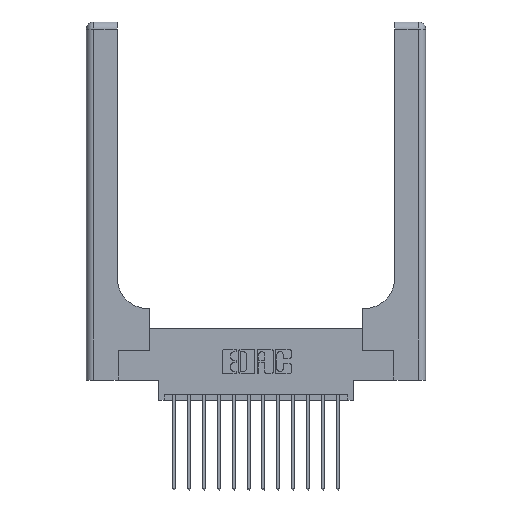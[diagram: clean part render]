
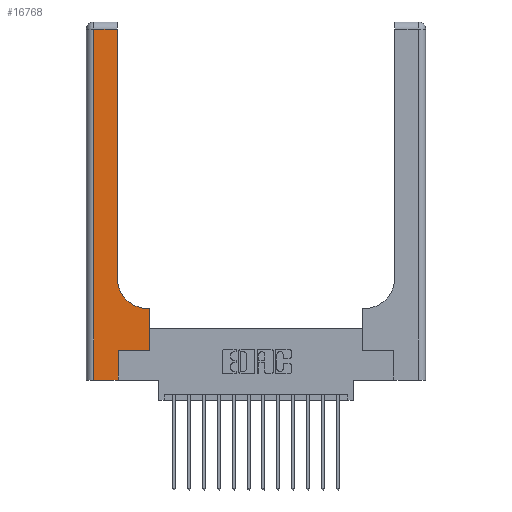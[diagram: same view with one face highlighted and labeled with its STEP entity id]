
A CAD part, top view. The second image highlights one B-rep face of the part: STEP entity #16768.
In plain terms, the highlighted planar face has unit normal (0, 0, 1).
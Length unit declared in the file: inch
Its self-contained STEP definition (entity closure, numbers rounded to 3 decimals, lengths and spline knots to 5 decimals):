
#131 = ORIENTED_EDGE ( 'NONE', *, *, #15163, .T. ) ;
#193 = EDGE_CURVE ( 'NONE', #11702, #6847, #12634, .T. ) ;
#345 = CARTESIAN_POINT ( 'NONE',  ( 0.06, 2.94, 0.37 ) ) ;
#442 = VERTEX_POINT ( 'NONE', #16277 ) ;
#686 = AXIS2_PLACEMENT_3D ( 'NONE', #5466, #14808, #6824 ) ;
#1284 = DIRECTION ( 'NONE',  ( 0., -1., 0. ) ) ;
#1679 = EDGE_CURVE ( 'NONE', #14367, #16168, #5903, .T. ) ;
#2014 = VERTEX_POINT ( 'NONE', #16160 ) ;
#2059 = LINE ( 'NONE', #8484, #12275 ) ;
#2062 = DIRECTION ( 'NONE',  ( 1., 0., 0. ) ) ;
#2220 = LINE ( 'NONE', #6354, #8893 ) ;
#2367 = VECTOR ( 'NONE', #11329, 39.37008 ) ;
#2972 = ORIENTED_EDGE ( 'NONE', *, *, #1679, .T. ) ;
#3179 = ORIENTED_EDGE ( 'NONE', *, *, #9093, .T. ) ;
#4419 = EDGE_CURVE ( 'NONE', #2014, #442, #9104, .T. ) ;
#4531 = CARTESIAN_POINT ( 'NONE',  ( 0.528, 0.6, 0.37 ) ) ;
#4649 = EDGE_CURVE ( 'NONE', #9263, #7784, #2220, .T. ) ;
#5007 = DIRECTION ( 'NONE',  ( -1., 0., 0. ) ) ;
#5103 = DIRECTION ( 'NONE',  ( 0., 1., 0. ) ) ;
#5149 = DIRECTION ( 'NONE',  ( 0., 0., -1. ) ) ;
#5466 = CARTESIAN_POINT ( 'NONE',  ( 0.51, 0.85, 0.37 ) ) ;
#5903 = LINE ( 'NONE', #9807, #2367 ) ;
#5970 = VECTOR ( 'NONE', #2062, 39.37008 ) ;
#6139 = AXIS2_PLACEMENT_3D ( 'NONE', #9118, #5149, #14471 ) ;
#6353 = ORIENTED_EDGE ( 'NONE', *, *, #4649, .T. ) ;
#6354 = CARTESIAN_POINT ( 'NONE',  ( 0.26, 0.6, 0.37 ) ) ;
#6809 = ORIENTED_EDGE ( 'NONE', *, *, #7417, .T. ) ;
#6824 = DIRECTION ( 'NONE',  ( 1., 0., 0. ) ) ;
#6847 = VERTEX_POINT ( 'NONE', #7455 ) ;
#6997 = FACE_OUTER_BOUND ( 'NONE', #16017, .T. ) ;
#7417 = EDGE_CURVE ( 'NONE', #7784, #14367, #12775, .T. ) ;
#7455 = CARTESIAN_POINT ( 'NONE',  ( 0.06, 0., 0.37 ) ) ;
#7784 = VERTEX_POINT ( 'NONE', #14375 ) ;
#7912 = CARTESIAN_POINT ( 'NONE',  ( 0.26, 2.94, 0.37 ) ) ;
#8066 = VECTOR ( 'NONE', #11810, 39.37008 ) ;
#8262 = VECTOR ( 'NONE', #1284, 39.37008 ) ;
#8484 = CARTESIAN_POINT ( 'NONE',  ( 0., 2.94, 0.37 ) ) ;
#8893 = VECTOR ( 'NONE', #5007, 39.37008 ) ;
#8925 = VECTOR ( 'NONE', #5103, 39.37008 ) ;
#9093 = EDGE_CURVE ( 'NONE', #9215, #2014, #10233, .T. ) ;
#9104 = LINE ( 'NONE', #11392, #5970 ) ;
#9118 = CARTESIAN_POINT ( 'NONE',  ( 0., 3., 0.37 ) ) ;
#9122 = CARTESIAN_POINT ( 'NONE',  ( 0., 0., 0.37 ) ) ;
#9215 = VERTEX_POINT ( 'NONE', #10963 ) ;
#9256 = CARTESIAN_POINT ( 'NONE',  ( 0.06, 3., 0.37 ) ) ;
#9263 = VERTEX_POINT ( 'NONE', #4531 ) ;
#9807 = CARTESIAN_POINT ( 'NONE',  ( 0.26, 3., 0.37 ) ) ;
#10233 = LINE ( 'NONE', #11843, #16864 ) ;
#10448 = EDGE_CURVE ( 'NONE', #16168, #11702, #2059, .T. ) ;
#10963 = CARTESIAN_POINT ( 'NONE',  ( 0.265, 0., 0.37 ) ) ;
#11329 = DIRECTION ( 'NONE',  ( 0., 1., 0. ) ) ;
#11392 = CARTESIAN_POINT ( 'NONE',  ( 0.265, 0.25, 0.37 ) ) ;
#11645 = ORIENTED_EDGE ( 'NONE', *, *, #4419, .T. ) ;
#11702 = VERTEX_POINT ( 'NONE', #345 ) ;
#11810 = DIRECTION ( 'NONE',  ( 1., 0., 0. ) ) ;
#11843 = CARTESIAN_POINT ( 'NONE',  ( 0.265, 0., 0.37 ) ) ;
#12275 = VECTOR ( 'NONE', #12500, 39.37008 ) ;
#12467 = LINE ( 'NONE', #14429, #8925 ) ;
#12500 = DIRECTION ( 'NONE',  ( -1., 0., 0. ) ) ;
#12634 = LINE ( 'NONE', #9256, #8262 ) ;
#12775 = CIRCLE ( 'NONE', #686, 0.25 ) ;
#12784 = ORIENTED_EDGE ( 'NONE', *, *, #14578, .T. ) ;
#13133 = PLANE ( 'NONE',  #6139 ) ;
#13163 = DIRECTION ( 'NONE',  ( 0., 1., 0. ) ) ;
#14070 = ORIENTED_EDGE ( 'NONE', *, *, #193, .T. ) ;
#14367 = VERTEX_POINT ( 'NONE', #16635 ) ;
#14375 = CARTESIAN_POINT ( 'NONE',  ( 0.51, 0.6, 0.37 ) ) ;
#14429 = CARTESIAN_POINT ( 'NONE',  ( 0.528, 0.25, 0.37 ) ) ;
#14471 = DIRECTION ( 'NONE',  ( -1., 0., 0. ) ) ;
#14578 = EDGE_CURVE ( 'NONE', #442, #9263, #12467, .T. ) ;
#14808 = DIRECTION ( 'NONE',  ( 0., 0., -1. ) ) ;
#15147 = LINE ( 'NONE', #9122, #8066 ) ;
#15163 = EDGE_CURVE ( 'NONE', #6847, #9215, #15147, .T. ) ;
#16017 = EDGE_LOOP ( 'NONE', ( #2972, #16669, #14070, #131, #3179, #11645, #12784, #6353, #6809 ) ) ;
#16160 = CARTESIAN_POINT ( 'NONE',  ( 0.265, 0.25, 0.37 ) ) ;
#16168 = VERTEX_POINT ( 'NONE', #7912 ) ;
#16277 = CARTESIAN_POINT ( 'NONE',  ( 0.528, 0.25, 0.37 ) ) ;
#16635 = CARTESIAN_POINT ( 'NONE',  ( 0.26, 0.85, 0.37 ) ) ;
#16669 = ORIENTED_EDGE ( 'NONE', *, *, #10448, .T. ) ;
#16768 = ADVANCED_FACE ( 'NONE', ( #6997 ), #13133, .F. ) ;
#16864 = VECTOR ( 'NONE', #13163, 39.37008 ) ;
